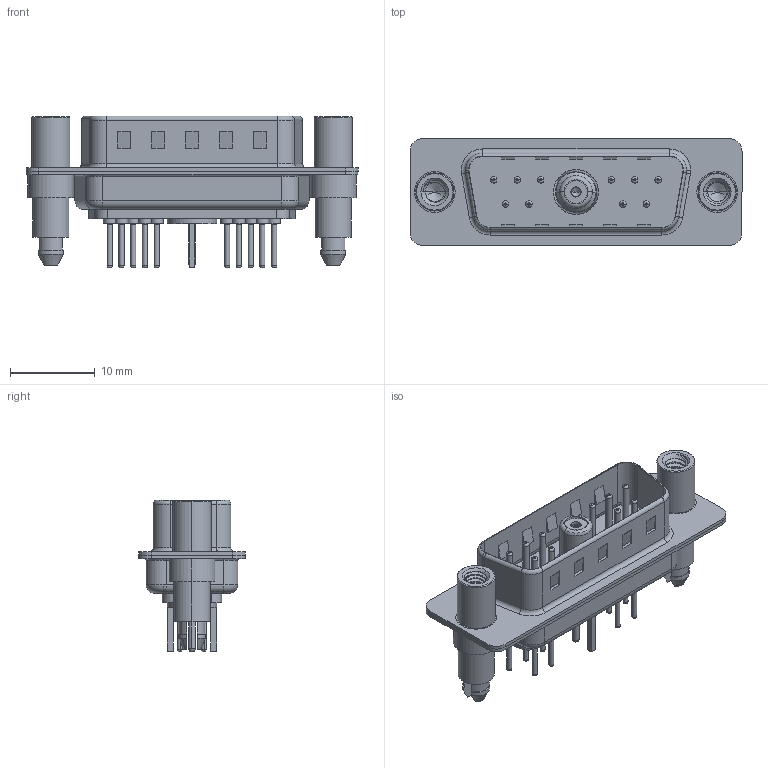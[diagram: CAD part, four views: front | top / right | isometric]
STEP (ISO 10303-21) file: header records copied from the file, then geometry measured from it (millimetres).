
FILE_DESCRIPTION (( 'STEP AP203' ), '1' );
FILE_NAME ('627-11W1224-5TE.STEP', '2019-05-25T13:39:43', ( '' ), ( '' ), 'SwSTEP 2.0', 'SolidWorks 2016', '' );
FILE_SCHEMA (( 'CONFIG_CONTROL_DESIGN' ));
Length unit declared in the file: millimetre
Products named in the file (14): Locking Collar; Socket_Str; 627Combo Housing_11W1; Co-Ax Jack Assy_S; 627Combo Shell Rear_15 Contacts; 627Combo Threaded Standoff and Boardlock_6; 627Combo Shell Front_15 Contacts; 627Combo Contact Row 1_24; 627Combo Threaded Standoff and Boardlock_E; 627Combo Contact Row 2_24; Co-Ax Jack_Straight PC Tail; 627-11W1224-5TE; Insulator Socket; Insulator Socket 2
Assembly tree (21 placements, depth 3):
  627-11W1224-5TE
    627Combo Housing_11W1
    627Combo Shell Rear_15 Contacts
    627Combo Shell Front_15 Contacts
    627Combo Threaded Standoff and Boardlock_E
    Co-Ax Jack Assy_S
      Co-Ax Jack_Straight PC Tail
      Insulator Socket
      Insulator Socket 2
      Locking Collar
      Socket_Str
    627Combo Threaded Standoff and Boardlock_6
    627Combo Contact Row 1_24  x6
    627Combo Contact Row 2_24  x4
Bounding box: 39.15 x 12.6 x 17.9 mm (x, y, z)
Volume: 2204.4 mm3; surface area: 5659.6 mm2
Topology: 20 solids, 23 shells, 889 faces, 2001 edges, 1233 vertices
Faces by surface type: cylinder 356, plane 283, torus 214, cone 26, bspline 8, sphere 2
Entity records: 23113 total; most frequent: CARTESIAN_POINT 5909, DIRECTION 3453, ORIENTED_EDGE 3086, EDGE_CURVE 1543, AXIS2_PLACEMENT_3D 1360, VERTEX_POINT 977, EDGE_LOOP 778, VECTOR 733
